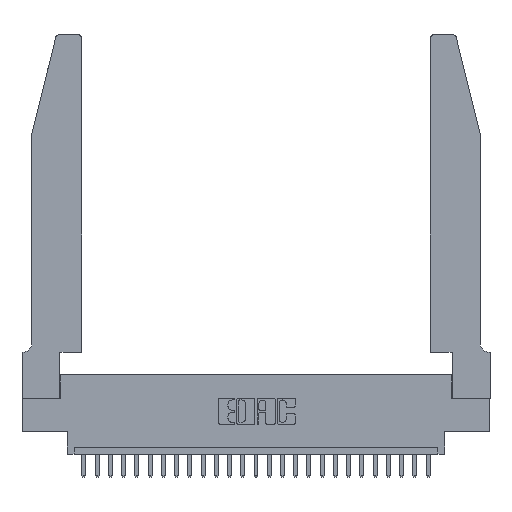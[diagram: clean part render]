
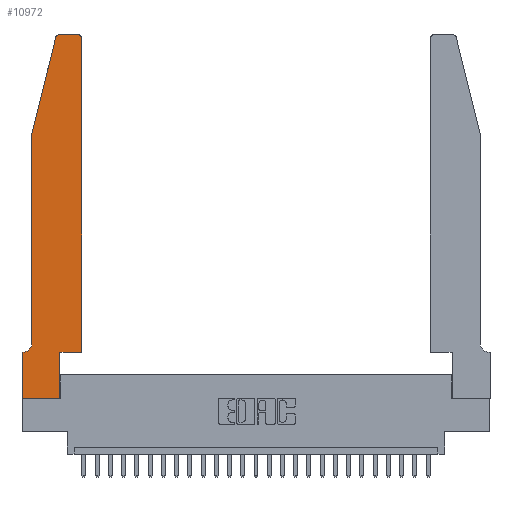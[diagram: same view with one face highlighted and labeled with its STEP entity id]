
A CAD part, top view. The second image highlights one B-rep face of the part: STEP entity #10972.
In plain terms, the highlighted planar face has unit normal (0, 0, 1).
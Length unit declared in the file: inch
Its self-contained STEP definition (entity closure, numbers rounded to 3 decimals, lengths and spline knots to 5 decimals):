
#93 = AXIS2_PLACEMENT_3D ( 'NONE', #23536, #251, #17506 ) ;
#186 = ORIENTED_EDGE ( 'NONE', *, *, #13498, .T. ) ;
#251 = DIRECTION ( 'NONE',  ( 0., 0., 1. ) ) ;
#1041 = DIRECTION ( 'NONE',  ( 0., -1., 0. ) ) ;
#1421 = VECTOR ( 'NONE', #5382, 39.37008 ) ;
#1563 = CARTESIAN_POINT ( 'NONE',  ( 0., 0.35, 0.37 ) ) ;
#1601 = LINE ( 'NONE', #14565, #27352 ) ;
#1750 = EDGE_CURVE ( 'NONE', #18351, #10848, #2088, .T. ) ;
#1894 = DIRECTION ( 'NONE',  ( 1., 0., 0. ) ) ;
#1985 = AXIS2_PLACEMENT_3D ( 'NONE', #4067, #25142, #12511 ) ;
#2012 = VERTEX_POINT ( 'NONE', #8767 ) ;
#2071 = DIRECTION ( 'NONE',  ( 0., 1., 0. ) ) ;
#2088 = LINE ( 'NONE', #7040, #1421 ) ;
#2184 = PLANE ( 'NONE',  #93 ) ;
#2361 = ORIENTED_EDGE ( 'NONE', *, *, #7498, .T. ) ;
#2837 = ORIENTED_EDGE ( 'NONE', *, *, #27360, .T. ) ;
#3681 = CARTESIAN_POINT ( 'NONE',  ( 0.0755, 0.42, 0.37 ) ) ;
#4033 = ORIENTED_EDGE ( 'NONE', *, *, #17654, .T. ) ;
#4063 = CARTESIAN_POINT ( 'NONE',  ( 0., 0., 0.37 ) ) ;
#4067 = CARTESIAN_POINT ( 'NONE',  ( 0.4205, 2.72, 0.37 ) ) ;
#4317 = DIRECTION ( 'NONE',  ( 0., 0., 1. ) ) ;
#4955 = VERTEX_POINT ( 'NONE', #5535 ) ;
#5171 = EDGE_CURVE ( 'NONE', #10848, #27321, #7018, .T. ) ;
#5325 = EDGE_LOOP ( 'NONE', ( #186, #4033, #16370, #2837, #24962, #22196, #16565, #7369, #15844, #9405, #22295, #2361 ) ) ;
#5382 = DIRECTION ( 'NONE',  ( 0., 1., 0. ) ) ;
#5535 = CARTESIAN_POINT ( 'NONE',  ( 0.0055, 0.35, 0.37 ) ) ;
#5659 = CARTESIAN_POINT ( 'NONE',  ( 0.4505, 0.35, 0.37 ) ) ;
#6073 = EDGE_CURVE ( 'NONE', #24262, #18033, #25475, .T. ) ;
#6208 = EDGE_CURVE ( 'NONE', #26367, #18351, #7631, .T. ) ;
#6262 = CARTESIAN_POINT ( 'NONE',  ( 0.2865, 0.35, 0.37 ) ) ;
#6303 = DIRECTION ( 'NONE',  ( 0., 0., -1. ) ) ;
#6373 = CARTESIAN_POINT ( 'NONE',  ( 0.284, 2.72, 0.37 ) ) ;
#6487 = CARTESIAN_POINT ( 'NONE',  ( 0.0055, 0.42, 0.37 ) ) ;
#6541 = CARTESIAN_POINT ( 'NONE',  ( 0.4205, 2.75, 0.37 ) ) ;
#6950 = AXIS2_PLACEMENT_3D ( 'NONE', #6373, #4317, #16635 ) ;
#7018 = LINE ( 'NONE', #20831, #12652 ) ;
#7027 = DIRECTION ( 'NONE',  ( 1., 0., 0. ) ) ;
#7040 = CARTESIAN_POINT ( 'NONE',  ( 0.2865, 0.35, 0.37 ) ) ;
#7279 = VECTOR ( 'NONE', #7027, 39.37008 ) ;
#7369 = ORIENTED_EDGE ( 'NONE', *, *, #6208, .T. ) ;
#7498 = EDGE_CURVE ( 'NONE', #2012, #21217, #17168, .T. ) ;
#7631 = LINE ( 'NONE', #4063, #7279 ) ;
#7951 = VECTOR ( 'NONE', #12507, 39.37008 ) ;
#8206 = CARTESIAN_POINT ( 'NONE',  ( 0., 0., 0.37 ) ) ;
#8625 = DIRECTION ( 'NONE',  ( -1., 0., 0. ) ) ;
#8767 = CARTESIAN_POINT ( 'NONE',  ( 0.4505, 2.72, 0.37 ) ) ;
#9405 = ORIENTED_EDGE ( 'NONE', *, *, #5171, .T. ) ;
#9536 = EDGE_CURVE ( 'NONE', #27321, #2012, #12769, .T. ) ;
#10312 = VECTOR ( 'NONE', #1041, 39.37008 ) ;
#10411 = EDGE_CURVE ( 'NONE', #4955, #16879, #13038, .T. ) ;
#10618 = CARTESIAN_POINT ( 'NONE',  ( 0.2865, 0., 0.37 ) ) ;
#10848 = VERTEX_POINT ( 'NONE', #6262 ) ;
#10941 = CARTESIAN_POINT ( 'NONE',  ( 0., 0., 0.37 ) ) ;
#10972 = ADVANCED_FACE ( 'NONE', ( #23918 ), #2184, .T. ) ;
#12057 = VECTOR ( 'NONE', #19940, 39.37008 ) ;
#12507 = DIRECTION ( 'NONE',  ( -0.239, -0.971, 0. ) ) ;
#12511 = DIRECTION ( 'NONE',  ( 1., 0., 0. ) ) ;
#12652 = VECTOR ( 'NONE', #1894, 39.37008 ) ;
#12769 = LINE ( 'NONE', #5659, #25646 ) ;
#13038 = LINE ( 'NONE', #26046, #12057 ) ;
#13498 = EDGE_CURVE ( 'NONE', #21217, #25853, #1601, .T. ) ;
#13999 = CARTESIAN_POINT ( 'NONE',  ( 0.0755, 2., 0.37 ) ) ;
#14565 = CARTESIAN_POINT ( 'NONE',  ( 0.2605, 2.75, 0.37 ) ) ;
#14740 = DIRECTION ( 'NONE',  ( -1., 0., 0. ) ) ;
#15844 = ORIENTED_EDGE ( 'NONE', *, *, #1750, .T. ) ;
#16347 = DIRECTION ( 'NONE',  ( 0., -1., 0. ) ) ;
#16370 = ORIENTED_EDGE ( 'NONE', *, *, #6073, .T. ) ;
#16494 = EDGE_CURVE ( 'NONE', #16879, #26367, #19981, .T. ) ;
#16565 = ORIENTED_EDGE ( 'NONE', *, *, #16494, .T. ) ;
#16635 = DIRECTION ( 'NONE',  ( 1., 0., 0. ) ) ;
#16879 = VERTEX_POINT ( 'NONE', #1563 ) ;
#17168 = CIRCLE ( 'NONE', #1985, 0.03 ) ;
#17506 = DIRECTION ( 'NONE',  ( 1., 0., 0. ) ) ;
#17544 = VERTEX_POINT ( 'NONE', #3681 ) ;
#17654 = EDGE_CURVE ( 'NONE', #25853, #24262, #21512, .T. ) ;
#18033 = VERTEX_POINT ( 'NONE', #19732 ) ;
#18351 = VERTEX_POINT ( 'NONE', #10618 ) ;
#18637 = CARTESIAN_POINT ( 'NONE',  ( 0.0755, 2., 0.37 ) ) ;
#19041 = EDGE_CURVE ( 'NONE', #17544, #4955, #22407, .T. ) ;
#19732 = CARTESIAN_POINT ( 'NONE',  ( 0.0755, 2., 0.37 ) ) ;
#19868 = LINE ( 'NONE', #13999, #10312 ) ;
#19940 = DIRECTION ( 'NONE',  ( -1., 0., 0. ) ) ;
#19981 = LINE ( 'NONE', #8206, #22290 ) ;
#20831 = CARTESIAN_POINT ( 'NONE',  ( 0.4505, 0.35, 0.37 ) ) ;
#21217 = VERTEX_POINT ( 'NONE', #6541 ) ;
#21512 = CIRCLE ( 'NONE', #6950, 0.03 ) ;
#22196 = ORIENTED_EDGE ( 'NONE', *, *, #10411, .T. ) ;
#22290 = VECTOR ( 'NONE', #16347, 39.37008 ) ;
#22295 = ORIENTED_EDGE ( 'NONE', *, *, #9536, .T. ) ;
#22299 = CARTESIAN_POINT ( 'NONE',  ( 0.4505, 0.35, 0.37 ) ) ;
#22407 = CIRCLE ( 'NONE', #24660, 0.07 ) ;
#23067 = CARTESIAN_POINT ( 'NONE',  ( 0.25487, 2.72718, 0.37 ) ) ;
#23536 = CARTESIAN_POINT ( 'NONE',  ( 0., 0.35, 0.37 ) ) ;
#23918 = FACE_OUTER_BOUND ( 'NONE', #5325, .T. ) ;
#24262 = VERTEX_POINT ( 'NONE', #23067 ) ;
#24660 = AXIS2_PLACEMENT_3D ( 'NONE', #6487, #6303, #8625 ) ;
#24811 = CARTESIAN_POINT ( 'NONE',  ( 0.284, 2.75, 0.37 ) ) ;
#24962 = ORIENTED_EDGE ( 'NONE', *, *, #19041, .T. ) ;
#25142 = DIRECTION ( 'NONE',  ( 0., 0., 1. ) ) ;
#25475 = LINE ( 'NONE', #18637, #7951 ) ;
#25646 = VECTOR ( 'NONE', #2071, 39.37008 ) ;
#25853 = VERTEX_POINT ( 'NONE', #24811 ) ;
#26046 = CARTESIAN_POINT ( 'NONE',  ( 0.0755, 0.35, 0.37 ) ) ;
#26367 = VERTEX_POINT ( 'NONE', #10941 ) ;
#27321 = VERTEX_POINT ( 'NONE', #22299 ) ;
#27352 = VECTOR ( 'NONE', #14740, 39.37008 ) ;
#27360 = EDGE_CURVE ( 'NONE', #18033, #17544, #19868, .T. ) ;
